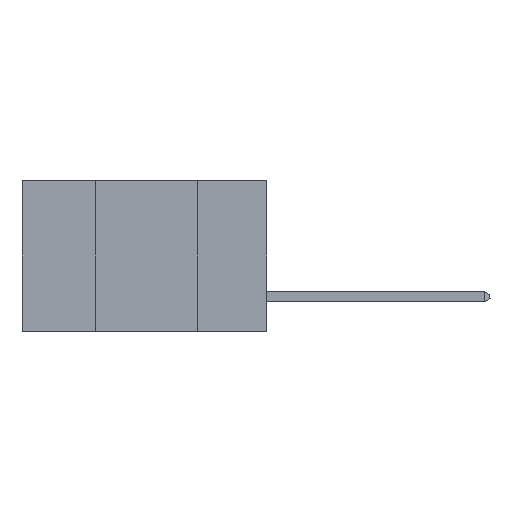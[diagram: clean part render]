
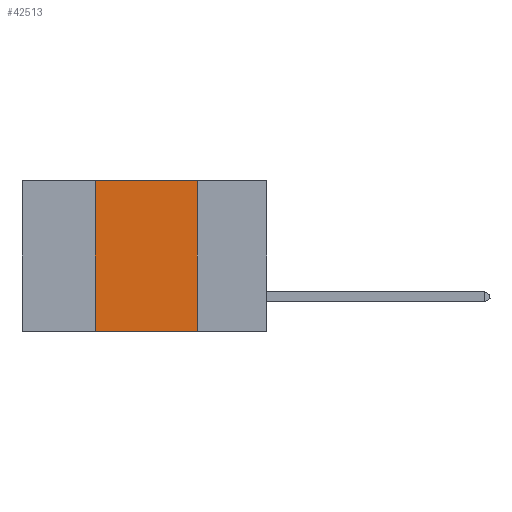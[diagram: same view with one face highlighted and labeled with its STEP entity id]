
A CAD part, left-side view. The second image highlights one B-rep face of the part: STEP entity #42513.
In plain terms, the highlighted planar face has unit normal (-1, 0, 0).
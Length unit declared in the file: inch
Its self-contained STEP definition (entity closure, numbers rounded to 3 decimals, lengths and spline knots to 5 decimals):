
#1183 = VERTEX_POINT ( 'NONE', #48364 ) ;
#1646 = EDGE_LOOP ( 'NONE', ( #8177, #47375, #3302, #45454 ) ) ;
#2187 = DIRECTION ( 'NONE',  ( 1., 0., 0. ) ) ;
#3008 = LINE ( 'NONE', #15258, #41041 ) ;
#3302 = ORIENTED_EDGE ( 'NONE', *, *, #27945, .F. ) ;
#8177 = ORIENTED_EDGE ( 'NONE', *, *, #47337, .F. ) ;
#9725 = CARTESIAN_POINT ( 'NONE',  ( 0., 0.17, 0. ) ) ;
#10130 = CARTESIAN_POINT ( 'NONE',  ( 0., 0.6, 0. ) ) ;
#11515 = CARTESIAN_POINT ( 'NONE',  ( 0., 0.17, 0. ) ) ;
#13004 = LINE ( 'NONE', #9725, #32604 ) ;
#13145 = DIRECTION ( 'NONE',  ( 0., -1., 0. ) ) ;
#13414 = LINE ( 'NONE', #32821, #32890 ) ;
#15258 = CARTESIAN_POINT ( 'NONE',  ( 0., 0.42, 0. ) ) ;
#15675 = VECTOR ( 'NONE', #33923, 39.37008 ) ;
#17505 = PLANE ( 'NONE',  #19379 ) ;
#19035 = CARTESIAN_POINT ( 'NONE',  ( 0., 0.17, -0.37 ) ) ;
#19379 = AXIS2_PLACEMENT_3D ( 'NONE', #10130, #2187, #21236 ) ;
#21236 = DIRECTION ( 'NONE',  ( 0., 0., -1. ) ) ;
#22520 = VERTEX_POINT ( 'NONE', #39494 ) ;
#23047 = EDGE_CURVE ( 'NONE', #22520, #25977, #13414, .T. ) ;
#25977 = VERTEX_POINT ( 'NONE', #11515 ) ;
#27945 = EDGE_CURVE ( 'NONE', #1183, #22520, #3008, .T. ) ;
#28543 = FACE_OUTER_BOUND ( 'NONE', #1646, .T. ) ;
#29393 = DIRECTION ( 'NONE',  ( 0., 0., -1. ) ) ;
#32604 = VECTOR ( 'NONE', #29393, 39.37008 ) ;
#32821 = CARTESIAN_POINT ( 'NONE',  ( 0., 0.6, 0. ) ) ;
#32890 = VECTOR ( 'NONE', #13145, 39.37008 ) ;
#33398 = LINE ( 'NONE', #45961, #15675 ) ;
#33923 = DIRECTION ( 'NONE',  ( 0., -1., 0. ) ) ;
#33972 = VERTEX_POINT ( 'NONE', #19035 ) ;
#39494 = CARTESIAN_POINT ( 'NONE',  ( 0., 0.42, 0. ) ) ;
#41041 = VECTOR ( 'NONE', #42700, 39.37008 ) ;
#42513 = ADVANCED_FACE ( 'NONE', ( #28543 ), #17505, .F. ) ;
#42700 = DIRECTION ( 'NONE',  ( 0., 0., 1. ) ) ;
#45454 = ORIENTED_EDGE ( 'NONE', *, *, #50506, .T. ) ;
#45961 = CARTESIAN_POINT ( 'NONE',  ( 0., 0.6, -0.37 ) ) ;
#47337 = EDGE_CURVE ( 'NONE', #25977, #33972, #13004, .T. ) ;
#47375 = ORIENTED_EDGE ( 'NONE', *, *, #23047, .F. ) ;
#48364 = CARTESIAN_POINT ( 'NONE',  ( 0., 0.42, -0.37 ) ) ;
#50506 = EDGE_CURVE ( 'NONE', #1183, #33972, #33398, .T. ) ;
